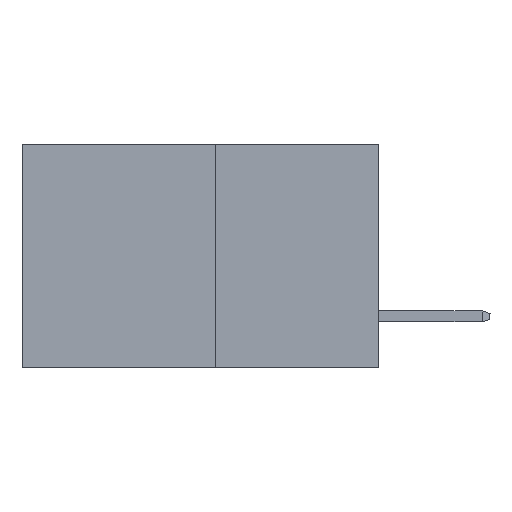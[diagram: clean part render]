
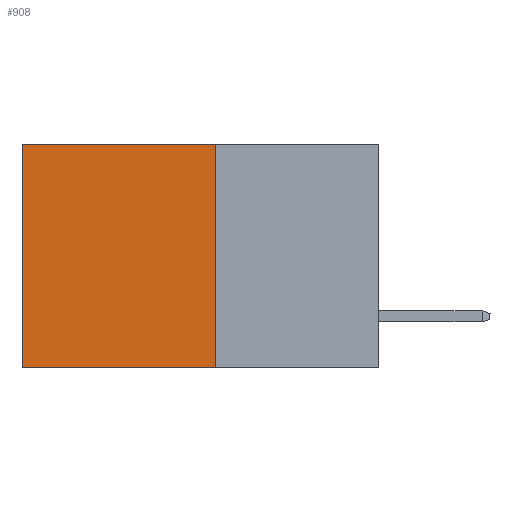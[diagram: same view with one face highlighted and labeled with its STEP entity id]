
A CAD part, left-side view. The second image highlights one B-rep face of the part: STEP entity #908.
In plain terms, the highlighted planar face has unit normal (-1, 0, 0).
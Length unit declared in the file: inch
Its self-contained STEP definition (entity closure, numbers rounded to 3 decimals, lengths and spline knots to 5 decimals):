
#869 = EDGE_CURVE ( 'NONE', #7588, #4875, #10236, .T. ) ;
#908 = ADVANCED_FACE ( 'NONE', ( #9186 ), #1107, .F. ) ;
#1107 = PLANE ( 'NONE',  #5527 ) ;
#1701 = DIRECTION ( 'NONE',  ( 0., 0., -1. ) ) ;
#2150 = CARTESIAN_POINT ( 'NONE',  ( 0.277, 0.27, -0.37 ) ) ;
#2179 = VECTOR ( 'NONE', #9341, 39.37008 ) ;
#3839 = CARTESIAN_POINT ( 'NONE',  ( 0.277, 0.27, -0.37 ) ) ;
#3924 = CARTESIAN_POINT ( 'NONE',  ( 0.277, 0.27, 0. ) ) ;
#4034 = VERTEX_POINT ( 'NONE', #13509 ) ;
#4875 = VERTEX_POINT ( 'NONE', #9427 ) ;
#5527 = AXIS2_PLACEMENT_3D ( 'NONE', #7623, #10954, #10783 ) ;
#5639 = EDGE_LOOP ( 'NONE', ( #7744, #7763, #7833, #7850 ) ) ;
#5859 = LINE ( 'NONE', #2150, #2179 ) ;
#6183 = VERTEX_POINT ( 'NONE', #11091 ) ;
#6460 = CARTESIAN_POINT ( 'NONE',  ( 0.277, 0.27, 0. ) ) ;
#7138 = VECTOR ( 'NONE', #14282, 39.37008 ) ;
#7588 = VERTEX_POINT ( 'NONE', #3924 ) ;
#7623 = CARTESIAN_POINT ( 'NONE',  ( 0.277, 0.27, -0.37 ) ) ;
#7744 = ORIENTED_EDGE ( 'NONE', *, *, #10752, .T. ) ;
#7763 = ORIENTED_EDGE ( 'NONE', *, *, #8172, .F. ) ;
#7833 = ORIENTED_EDGE ( 'NONE', *, *, #8428, .F. ) ;
#7850 = ORIENTED_EDGE ( 'NONE', *, *, #869, .T. ) ;
#8172 = EDGE_CURVE ( 'NONE', #4034, #6183, #10187, .T. ) ;
#8428 = EDGE_CURVE ( 'NONE', #7588, #4034, #5859, .T. ) ;
#9186 = FACE_OUTER_BOUND ( 'NONE', #5639, .T. ) ;
#9341 = DIRECTION ( 'NONE',  ( 0., 0., -1. ) ) ;
#9427 = CARTESIAN_POINT ( 'NONE',  ( 0.277, 0.59, 0. ) ) ;
#9584 = DIRECTION ( 'NONE',  ( 0., 1., 0. ) ) ;
#10187 = LINE ( 'NONE', #3839, #7138 ) ;
#10236 = LINE ( 'NONE', #6460, #12904 ) ;
#10752 = EDGE_CURVE ( 'NONE', #4875, #6183, #12996, .T. ) ;
#10783 = DIRECTION ( 'NONE',  ( 0., 0., -1. ) ) ;
#10954 = DIRECTION ( 'NONE',  ( 1., 0., 0. ) ) ;
#11091 = CARTESIAN_POINT ( 'NONE',  ( 0.277, 0.59, -0.37 ) ) ;
#12904 = VECTOR ( 'NONE', #9584, 39.37008 ) ;
#12996 = LINE ( 'NONE', #13457, #15226 ) ;
#13457 = CARTESIAN_POINT ( 'NONE',  ( 0.277, 0.59, -0.37 ) ) ;
#13509 = CARTESIAN_POINT ( 'NONE',  ( 0.277, 0.27, -0.37 ) ) ;
#14282 = DIRECTION ( 'NONE',  ( 0., 1., 0. ) ) ;
#15226 = VECTOR ( 'NONE', #1701, 39.37008 ) ;
